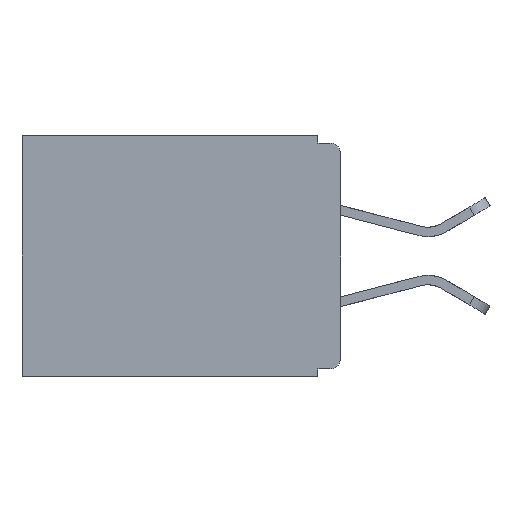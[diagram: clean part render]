
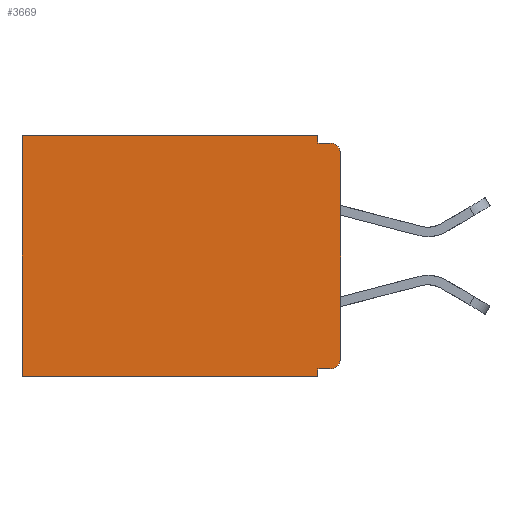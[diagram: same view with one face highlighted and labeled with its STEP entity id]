
A CAD part, left-side view. The second image highlights one B-rep face of the part: STEP entity #3669.
In plain terms, the highlighted planar face has unit normal (-1, 0, 0).
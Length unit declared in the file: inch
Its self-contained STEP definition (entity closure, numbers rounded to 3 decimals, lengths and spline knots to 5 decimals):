
#91 = VECTOR ( 'NONE', #6275, 39.37008 ) ;
#540 = ORIENTED_EDGE ( 'NONE', *, *, #3591, .F. ) ;
#805 = ORIENTED_EDGE ( 'NONE', *, *, #5697, .F. ) ;
#935 = ORIENTED_EDGE ( 'NONE', *, *, #12032, .T. ) ;
#1593 = DIRECTION ( 'NONE',  ( 0., 0., -1. ) ) ;
#1896 = VERTEX_POINT ( 'NONE', #8494 ) ;
#1936 = DIRECTION ( 'NONE',  ( 0., 0., -1. ) ) ;
#2205 = DIRECTION ( 'NONE',  ( 0., 1., 0. ) ) ;
#2909 = LINE ( 'NONE', #12353, #7179 ) ;
#3395 = ORIENTED_EDGE ( 'NONE', *, *, #5300, .F. ) ;
#3591 = EDGE_CURVE ( 'NONE', #1896, #8684, #14928, .T. ) ;
#3669 = ADVANCED_FACE ( 'NONE', ( #16676 ), #16950, .F. ) ;
#3715 = CARTESIAN_POINT ( 'NONE',  ( 0.3, 0., -0.33 ) ) ;
#3869 = CARTESIAN_POINT ( 'NONE',  ( 0.3, 0.031, -0.33 ) ) ;
#4090 = VECTOR ( 'NONE', #8274, 39.37008 ) ;
#4608 = ORIENTED_EDGE ( 'NONE', *, *, #17467, .T. ) ;
#4648 = LINE ( 'NONE', #5327, #12829 ) ;
#5011 = CARTESIAN_POINT ( 'NONE',  ( 0.3, 0.031, 0. ) ) ;
#5143 = LINE ( 'NONE', #5011, #14825 ) ;
#5150 = EDGE_CURVE ( 'NONE', #9537, #10607, #2909, .T. ) ;
#5300 = EDGE_CURVE ( 'NONE', #8684, #12547, #4648, .T. ) ;
#5327 = CARTESIAN_POINT ( 'NONE',  ( 0.3, 0., -0.33 ) ) ;
#5368 = CARTESIAN_POINT ( 'NONE',  ( 0.3, 0.437, -0.33 ) ) ;
#5597 = DIRECTION ( 'NONE',  ( 0., 1., 0. ) ) ;
#5697 = EDGE_CURVE ( 'NONE', #9537, #7830, #5143, .T. ) ;
#5723 = DIRECTION ( 'NONE',  ( 0., 0., -1. ) ) ;
#6275 = DIRECTION ( 'NONE',  ( 0., -1., 0. ) ) ;
#6377 = ORIENTED_EDGE ( 'NONE', *, *, #13850, .F. ) ;
#6931 = DIRECTION ( 'NONE',  ( 1., 0., 0. ) ) ;
#6986 = EDGE_CURVE ( 'NONE', #15469, #12189, #17488, .T. ) ;
#7018 = CARTESIAN_POINT ( 'NONE',  ( 0.3, 0., -0.32 ) ) ;
#7179 = VECTOR ( 'NONE', #18553, 39.37008 ) ;
#7450 = CARTESIAN_POINT ( 'NONE',  ( 0.3, 0.015, -0.305 ) ) ;
#7830 = VERTEX_POINT ( 'NONE', #19027 ) ;
#8075 = VERTEX_POINT ( 'NONE', #14601 ) ;
#8274 = DIRECTION ( 'NONE',  ( 0., 0., -1. ) ) ;
#8494 = CARTESIAN_POINT ( 'NONE',  ( 0.3, 0.031, -0.32 ) ) ;
#8684 = VERTEX_POINT ( 'NONE', #3869 ) ;
#9075 = DIRECTION ( 'NONE',  ( 0., 0., -1. ) ) ;
#9163 = LINE ( 'NONE', #16030, #91 ) ;
#9537 = VERTEX_POINT ( 'NONE', #20035 ) ;
#9869 = EDGE_CURVE ( 'NONE', #15469, #11628, #17604, .T. ) ;
#10283 = VECTOR ( 'NONE', #2205, 39.37008 ) ;
#10607 = VERTEX_POINT ( 'NONE', #11537 ) ;
#11276 = DIRECTION ( 'NONE',  ( -1., 0., 0. ) ) ;
#11537 = CARTESIAN_POINT ( 'NONE',  ( 0.3, 0.437, 0. ) ) ;
#11628 = VERTEX_POINT ( 'NONE', #14184 ) ;
#12032 = EDGE_CURVE ( 'NONE', #8075, #12189, #15562, .T. ) ;
#12189 = VERTEX_POINT ( 'NONE', #19035 ) ;
#12353 = CARTESIAN_POINT ( 'NONE',  ( 0.3, 0., 0. ) ) ;
#12547 = VERTEX_POINT ( 'NONE', #5368 ) ;
#12754 = LINE ( 'NONE', #19558, #4090 ) ;
#12829 = VECTOR ( 'NONE', #5597, 39.37008 ) ;
#13224 = CARTESIAN_POINT ( 'NONE',  ( 0.3, 0., -0.33 ) ) ;
#13696 = AXIS2_PLACEMENT_3D ( 'NONE', #7450, #18750, #9075 ) ;
#13850 = EDGE_CURVE ( 'NONE', #8075, #1896, #15146, .T. ) ;
#14184 = CARTESIAN_POINT ( 'NONE',  ( 0.3, 0.015, -0.01 ) ) ;
#14438 = VECTOR ( 'NONE', #5723, 39.37008 ) ;
#14601 = CARTESIAN_POINT ( 'NONE',  ( 0.3, 0.015, -0.32 ) ) ;
#14825 = VECTOR ( 'NONE', #1936, 39.37008 ) ;
#14928 = LINE ( 'NONE', #18563, #14438 ) ;
#15048 = ORIENTED_EDGE ( 'NONE', *, *, #5150, .T. ) ;
#15146 = LINE ( 'NONE', #7018, #10283 ) ;
#15469 = VERTEX_POINT ( 'NONE', #15718 ) ;
#15562 = CIRCLE ( 'NONE', #13696, 0.015 ) ;
#15718 = CARTESIAN_POINT ( 'NONE',  ( 0.3, 0., -0.025 ) ) ;
#16030 = CARTESIAN_POINT ( 'NONE',  ( 0.3, 0., -0.01 ) ) ;
#16676 = FACE_OUTER_BOUND ( 'NONE', #20343, .T. ) ;
#16807 = EDGE_CURVE ( 'NONE', #7830, #11628, #9163, .T. ) ;
#16950 = PLANE ( 'NONE',  #18549 ) ;
#16985 = VECTOR ( 'NONE', #17961, 39.37008 ) ;
#17467 = EDGE_CURVE ( 'NONE', #10607, #12547, #12754, .T. ) ;
#17488 = LINE ( 'NONE', #13224, #16985 ) ;
#17538 = DIRECTION ( 'NONE',  ( 0., 0., -1. ) ) ;
#17604 = CIRCLE ( 'NONE', #20015, 0.015 ) ;
#17961 = DIRECTION ( 'NONE',  ( 0., 0., -1. ) ) ;
#18549 = AXIS2_PLACEMENT_3D ( 'NONE', #3715, #6931, #17538 ) ;
#18553 = DIRECTION ( 'NONE',  ( 0., 1., 0. ) ) ;
#18563 = CARTESIAN_POINT ( 'NONE',  ( 0.3, 0.031, -0.33 ) ) ;
#18750 = DIRECTION ( 'NONE',  ( -1., 0., 0. ) ) ;
#18758 = ORIENTED_EDGE ( 'NONE', *, *, #9869, .T. ) ;
#18839 = ORIENTED_EDGE ( 'NONE', *, *, #16807, .F. ) ;
#18988 = ORIENTED_EDGE ( 'NONE', *, *, #6986, .F. ) ;
#19027 = CARTESIAN_POINT ( 'NONE',  ( 0.3, 0.031, -0.01 ) ) ;
#19035 = CARTESIAN_POINT ( 'NONE',  ( 0.3, 0., -0.305 ) ) ;
#19558 = CARTESIAN_POINT ( 'NONE',  ( 0.3, 0.437, -0.33 ) ) ;
#20015 = AXIS2_PLACEMENT_3D ( 'NONE', #20817, #11276, #1593 ) ;
#20035 = CARTESIAN_POINT ( 'NONE',  ( 0.3, 0.031, 0. ) ) ;
#20343 = EDGE_LOOP ( 'NONE', ( #18988, #18758, #18839, #805, #15048, #4608, #3395, #540, #6377, #935 ) ) ;
#20817 = CARTESIAN_POINT ( 'NONE',  ( 0.3, 0.015, -0.025 ) ) ;
